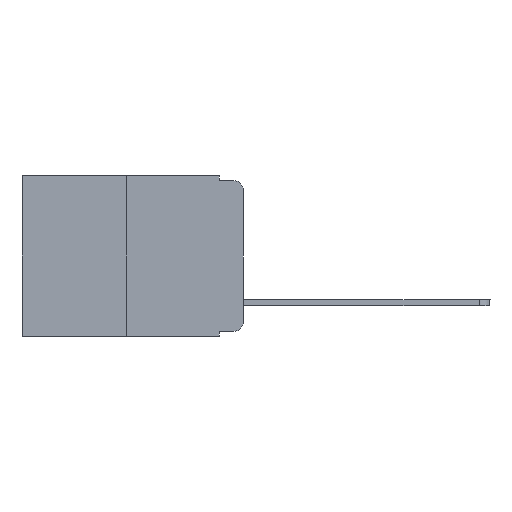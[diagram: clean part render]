
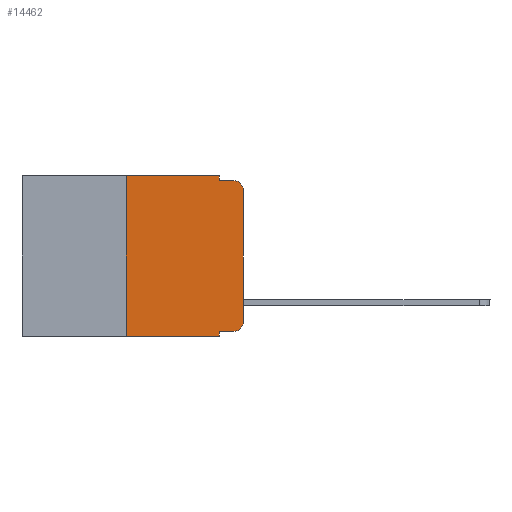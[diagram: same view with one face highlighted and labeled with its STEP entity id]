
A CAD part, left-side view. The second image highlights one B-rep face of the part: STEP entity #14462.
In plain terms, the highlighted planar face has unit normal (-1, 0, 0).
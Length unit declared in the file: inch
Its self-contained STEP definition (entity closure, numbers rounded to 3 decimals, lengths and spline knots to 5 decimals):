
#271 = DIRECTION ( 'NONE',  ( -1., 0., 0. ) ) ;
#732 = CARTESIAN_POINT ( 'NONE',  ( 0., 0.473, 0. ) ) ;
#749 = CARTESIAN_POINT ( 'NONE',  ( 0., 0.051, -0.01 ) ) ;
#926 = VECTOR ( 'NONE', #16273, 39.37008 ) ;
#1234 = VERTEX_POINT ( 'NONE', #10461 ) ;
#1847 = VERTEX_POINT ( 'NONE', #11458 ) ;
#1858 = LINE ( 'NONE', #9771, #20094 ) ;
#1988 = EDGE_LOOP ( 'NONE', ( #6696, #3136, #16380, #11618, #23413, #10047, #5491, #6918, #22756, #3074 ) ) ;
#2030 = CARTESIAN_POINT ( 'NONE',  ( 0., 0.25, 0. ) ) ;
#3074 = ORIENTED_EDGE ( 'NONE', *, *, #13089, .T. ) ;
#3136 = ORIENTED_EDGE ( 'NONE', *, *, #25822, .T. ) ;
#3365 = VECTOR ( 'NONE', #12128, 39.37008 ) ;
#3638 = LINE ( 'NONE', #15167, #25997 ) ;
#3653 = CARTESIAN_POINT ( 'NONE',  ( 0., 0.051, 0. ) ) ;
#4149 = CARTESIAN_POINT ( 'NONE',  ( 0., 0.051, 0. ) ) ;
#4798 = DIRECTION ( 'NONE',  ( 0., -1., 0. ) ) ;
#5255 = LINE ( 'NONE', #749, #24735 ) ;
#5490 = CARTESIAN_POINT ( 'NONE',  ( 0., 0., -0.03 ) ) ;
#5491 = ORIENTED_EDGE ( 'NONE', *, *, #19673, .T. ) ;
#5644 = DIRECTION ( 'NONE',  ( 0., 0., -1. ) ) ;
#5668 = DIRECTION ( 'NONE',  ( 0., 0., -1. ) ) ;
#5777 = CIRCLE ( 'NONE', #25654, 0.02 ) ;
#6696 = ORIENTED_EDGE ( 'NONE', *, *, #9729, .T. ) ;
#6753 = PLANE ( 'NONE',  #25619 ) ;
#6918 = ORIENTED_EDGE ( 'NONE', *, *, #21221, .F. ) ;
#6936 = DIRECTION ( 'NONE',  ( 0., 0., -1. ) ) ;
#8083 = VECTOR ( 'NONE', #18769, 39.37008 ) ;
#8118 = VERTEX_POINT ( 'NONE', #24489 ) ;
#8695 = DIRECTION ( 'NONE',  ( 0., -1., 0. ) ) ;
#8778 = CARTESIAN_POINT ( 'NONE',  ( 0., 0.25, 0. ) ) ;
#9037 = DIRECTION ( 'NONE',  ( 1., 0., 0. ) ) ;
#9040 = DIRECTION ( 'NONE',  ( 0., 0., 1. ) ) ;
#9729 = EDGE_CURVE ( 'NONE', #1847, #16598, #14044, .T. ) ;
#9771 = CARTESIAN_POINT ( 'NONE',  ( 0., 0.473, -0.343 ) ) ;
#10047 = ORIENTED_EDGE ( 'NONE', *, *, #11297, .F. ) ;
#10126 = CARTESIAN_POINT ( 'NONE',  ( 0., 0., 0. ) ) ;
#10363 = LINE ( 'NONE', #3653, #15395 ) ;
#10461 = CARTESIAN_POINT ( 'NONE',  ( 0., 0.051, 0. ) ) ;
#10679 = VERTEX_POINT ( 'NONE', #22588 ) ;
#11297 = EDGE_CURVE ( 'NONE', #15333, #13561, #20519, .T. ) ;
#11387 = LINE ( 'NONE', #4149, #926 ) ;
#11458 = CARTESIAN_POINT ( 'NONE',  ( 0., 0., -0.313 ) ) ;
#11618 = ORIENTED_EDGE ( 'NONE', *, *, #13528, .F. ) ;
#12128 = DIRECTION ( 'NONE',  ( 0., 0., 1. ) ) ;
#13089 = EDGE_CURVE ( 'NONE', #13180, #1847, #14800, .T. ) ;
#13180 = VERTEX_POINT ( 'NONE', #16393 ) ;
#13528 = EDGE_CURVE ( 'NONE', #1234, #8118, #10363, .T. ) ;
#13561 = VERTEX_POINT ( 'NONE', #2030 ) ;
#14044 = LINE ( 'NONE', #10126, #3365 ) ;
#14390 = FACE_OUTER_BOUND ( 'NONE', #1988, .T. ) ;
#14462 = ADVANCED_FACE ( 'NONE', ( #14390 ), #6753, .F. ) ;
#14575 = EDGE_CURVE ( 'NONE', #10679, #13180, #17535, .T. ) ;
#14800 = CIRCLE ( 'NONE', #21816, 0.02 ) ;
#15167 = CARTESIAN_POINT ( 'NONE',  ( 0., 0.473, 0. ) ) ;
#15222 = CARTESIAN_POINT ( 'NONE',  ( 0., 0.051, -0.343 ) ) ;
#15333 = VERTEX_POINT ( 'NONE', #22008 ) ;
#15395 = VECTOR ( 'NONE', #5668, 39.37008 ) ;
#15839 = VECTOR ( 'NONE', #9040, 39.37008 ) ;
#16273 = DIRECTION ( 'NONE',  ( 0., 0., -1. ) ) ;
#16315 = DIRECTION ( 'NONE',  ( 0., 0., -1. ) ) ;
#16380 = ORIENTED_EDGE ( 'NONE', *, *, #24263, .F. ) ;
#16393 = CARTESIAN_POINT ( 'NONE',  ( 0., 0.02, -0.333 ) ) ;
#16598 = VERTEX_POINT ( 'NONE', #5490 ) ;
#17535 = LINE ( 'NONE', #23188, #8083 ) ;
#17680 = CARTESIAN_POINT ( 'NONE',  ( 0., 0.02, -0.03 ) ) ;
#18402 = CARTESIAN_POINT ( 'NONE',  ( 0., 0.02, -0.313 ) ) ;
#18769 = DIRECTION ( 'NONE',  ( 0., -1., 0. ) ) ;
#19449 = VERTEX_POINT ( 'NONE', #15222 ) ;
#19673 = EDGE_CURVE ( 'NONE', #15333, #19449, #1858, .T. ) ;
#20094 = VECTOR ( 'NONE', #26070, 39.37008 ) ;
#20519 = LINE ( 'NONE', #8778, #15839 ) ;
#21221 = EDGE_CURVE ( 'NONE', #10679, #19449, #11387, .T. ) ;
#21816 = AXIS2_PLACEMENT_3D ( 'NONE', #18402, #271, #16315 ) ;
#22008 = CARTESIAN_POINT ( 'NONE',  ( 0., 0.25, -0.343 ) ) ;
#22588 = CARTESIAN_POINT ( 'NONE',  ( 0., 0.051, -0.333 ) ) ;
#22756 = ORIENTED_EDGE ( 'NONE', *, *, #14575, .T. ) ;
#22904 = CARTESIAN_POINT ( 'NONE',  ( 0., 0.02, -0.01 ) ) ;
#23188 = CARTESIAN_POINT ( 'NONE',  ( 0., 0.051, -0.333 ) ) ;
#23413 = ORIENTED_EDGE ( 'NONE', *, *, #24991, .F. ) ;
#24263 = EDGE_CURVE ( 'NONE', #8118, #26021, #5255, .T. ) ;
#24489 = CARTESIAN_POINT ( 'NONE',  ( 0., 0.051, -0.01 ) ) ;
#24735 = VECTOR ( 'NONE', #8695, 39.37008 ) ;
#24991 = EDGE_CURVE ( 'NONE', #13561, #1234, #3638, .T. ) ;
#25572 = DIRECTION ( 'NONE',  ( -1., 0., 0. ) ) ;
#25619 = AXIS2_PLACEMENT_3D ( 'NONE', #732, #9037, #6936 ) ;
#25654 = AXIS2_PLACEMENT_3D ( 'NONE', #17680, #25572, #5644 ) ;
#25822 = EDGE_CURVE ( 'NONE', #16598, #26021, #5777, .T. ) ;
#25997 = VECTOR ( 'NONE', #4798, 39.37008 ) ;
#26021 = VERTEX_POINT ( 'NONE', #22904 ) ;
#26070 = DIRECTION ( 'NONE',  ( 0., -1., 0. ) ) ;
